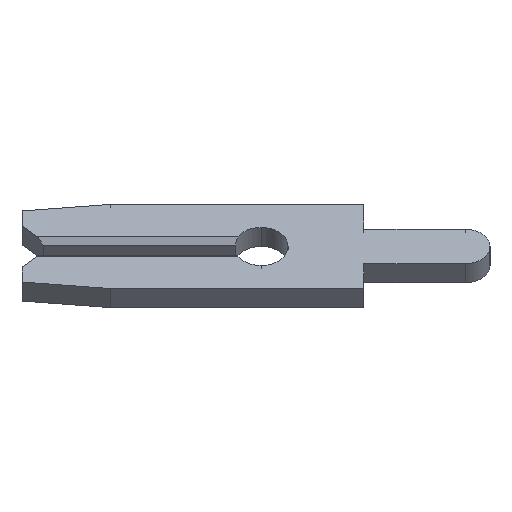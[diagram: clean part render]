
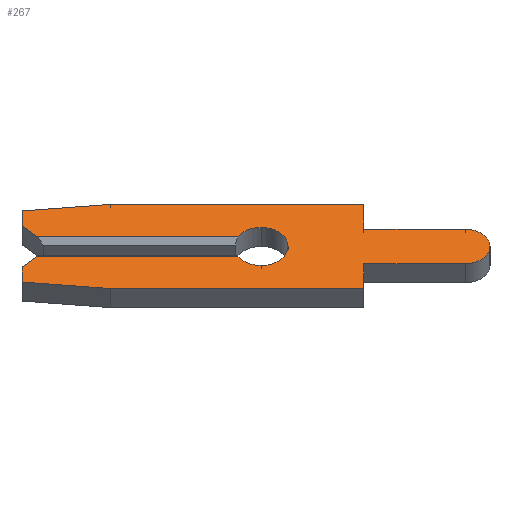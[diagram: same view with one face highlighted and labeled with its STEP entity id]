
A CAD part, left-side view. The second image highlights one B-rep face of the part: STEP entity #267.
In plain terms, the highlighted face is planar.
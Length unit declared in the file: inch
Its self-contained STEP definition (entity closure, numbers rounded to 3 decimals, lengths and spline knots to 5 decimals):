
#16 = EDGE_CURVE ( 'NONE', #715, #768, #471, .T. ) ;
#20 = DIRECTION ( 'NONE',  ( 0., 0., -1. ) ) ;
#25 = ORIENTED_EDGE ( 'NONE', *, *, #1155, .F. ) ;
#41 = CIRCLE ( 'NONE', #1211, 0.0235 ) ;
#47 = CARTESIAN_POINT ( 'NONE',  ( -0.013, 0., 0. ) ) ;
#56 = VECTOR ( 'NONE', #752, 39.37008 ) ;
#82 = ORIENTED_EDGE ( 'NONE', *, *, #520, .F. ) ;
#83 = VERTEX_POINT ( 'NONE', #694 ) ;
#90 = VERTEX_POINT ( 'NONE', #795 ) ;
#103 = VECTOR ( 'NONE', #990, 39.37008 ) ;
#115 = AXIS2_PLACEMENT_3D ( 'NONE', #521, #334, #530 ) ;
#136 = DIRECTION ( 'NONE',  ( 1., 0., 0. ) ) ;
#151 = EDGE_LOOP ( 'NONE', ( #186, #346, #287, #1049, #719, #270, #311, #524, #25, #552, #1169, #490, #344, #538, #629, #482, #82, #932 ) ) ;
#157 = EDGE_CURVE ( 'NONE', #233, #443, #610, .T. ) ;
#159 = VERTEX_POINT ( 'NONE', #923 ) ;
#168 = CIRCLE ( 'NONE', #907, 0.026 ) ;
#169 = AXIS2_PLACEMENT_3D ( 'NONE', #423, #1178, #20 ) ;
#186 = ORIENTED_EDGE ( 'NONE', *, *, #855, .T. ) ;
#187 = CARTESIAN_POINT ( 'NONE',  ( -0.013, -0.099, 0.0575 ) ) ;
#212 = CARTESIAN_POINT ( 'NONE',  ( -0.013, 0.146, -0.0575 ) ) ;
#213 = LINE ( 'NONE', #580, #922 ) ;
#221 = VERTEX_POINT ( 'NONE', #709 ) ;
#232 = DIRECTION ( 'NONE',  ( 0., -1., 0. ) ) ;
#233 = VERTEX_POINT ( 'NONE', #624 ) ;
#241 = VECTOR ( 'NONE', #620, 39.37008 ) ;
#261 = DIRECTION ( 'NONE',  ( -1., 0., 0. ) ) ;
#267 = ADVANCED_FACE ( 'NONE', ( #796 ), #823, .F. ) ;
#270 = ORIENTED_EDGE ( 'NONE', *, *, #1228, .F. ) ;
#276 = LINE ( 'NONE', #856, #56 ) ;
#287 = ORIENTED_EDGE ( 'NONE', *, *, #306, .F. ) ;
#294 = DIRECTION ( 'NONE',  ( 0., 0., 1. ) ) ;
#306 = EDGE_CURVE ( 'NONE', #369, #233, #168, .T. ) ;
#311 = ORIENTED_EDGE ( 'NONE', *, *, #755, .F. ) ;
#315 = VECTOR ( 'NONE', #906, 39.37008 ) ;
#334 = DIRECTION ( 'NONE',  ( -1., 0., 0. ) ) ;
#342 = CIRCLE ( 'NONE', #169, 0.026 ) ;
#344 = ORIENTED_EDGE ( 'NONE', *, *, #748, .F. ) ;
#346 = ORIENTED_EDGE ( 'NONE', *, *, #157, .F. ) ;
#348 = CARTESIAN_POINT ( 'NONE',  ( -0.013, 0.216, 0.013 ) ) ;
#363 = CARTESIAN_POINT ( 'NONE',  ( -0.013, 0.146, 0.0575 ) ) ;
#364 = LINE ( 'NONE', #685, #103 ) ;
#369 = VERTEX_POINT ( 'NONE', #827 ) ;
#374 = LINE ( 'NONE', #749, #789 ) ;
#379 = CARTESIAN_POINT ( 'NONE',  ( -0.013, 0.231, -0.04857 ) ) ;
#381 = DIRECTION ( 'NONE',  ( 0., 0.995, 0.105 ) ) ;
#395 = CARTESIAN_POINT ( 'NONE',  ( -0.013, -0.099, -0.0575 ) ) ;
#423 = CARTESIAN_POINT ( 'NONE',  ( -0.013, 0., 0. ) ) ;
#436 = EDGE_CURVE ( 'NONE', #810, #618, #509, .T. ) ;
#441 = EDGE_CURVE ( 'NONE', #159, #1137, #41, .T. ) ;
#443 = VERTEX_POINT ( 'NONE', #651 ) ;
#455 = DIRECTION ( 'NONE',  ( 0., -1., 0. ) ) ;
#457 = EDGE_CURVE ( 'NONE', #83, #688, #539, .T. ) ;
#467 = LINE ( 'NONE', #1205, #1192 ) ;
#471 = LINE ( 'NONE', #1003, #241 ) ;
#482 = ORIENTED_EDGE ( 'NONE', *, *, #998, .F. ) ;
#486 = CARTESIAN_POINT ( 'NONE',  ( -0.013, 0.2105, 0.0075 ) ) ;
#490 = ORIENTED_EDGE ( 'NONE', *, *, #441, .F. ) ;
#505 = VECTOR ( 'NONE', #381, 39.37008 ) ;
#509 = LINE ( 'NONE', #729, #1013 ) ;
#513 = CARTESIAN_POINT ( 'NONE',  ( -0.013, 0.231, 0.013 ) ) ;
#520 = EDGE_CURVE ( 'NONE', #1188, #90, #374, .T. ) ;
#521 = CARTESIAN_POINT ( 'NONE',  ( -0.013, 0., 0. ) ) ;
#524 = ORIENTED_EDGE ( 'NONE', *, *, #581, .F. ) ;
#530 = DIRECTION ( 'NONE',  ( 0., 0., -1. ) ) ;
#538 = ORIENTED_EDGE ( 'NONE', *, *, #1117, .F. ) ;
#539 = LINE ( 'NONE', #363, #984 ) ;
#540 = DIRECTION ( 'NONE',  ( 0., 1., 0. ) ) ;
#552 = ORIENTED_EDGE ( 'NONE', *, *, #16, .F. ) ;
#554 = VECTOR ( 'NONE', #1194, 39.37008 ) ;
#580 = CARTESIAN_POINT ( 'NONE',  ( -0.013, 0.231, -0.028 ) ) ;
#581 = EDGE_CURVE ( 'NONE', #738, #221, #645, .T. ) ;
#597 = DIRECTION ( 'NONE',  ( 0., 0.707, 0.707 ) ) ;
#610 = CIRCLE ( 'NONE', #115, 0.026 ) ;
#618 = VERTEX_POINT ( 'NONE', #949 ) ;
#620 = DIRECTION ( 'NONE',  ( 0., 0., -1. ) ) ;
#624 = CARTESIAN_POINT ( 'NONE',  ( -0.013, 0., 0.026 ) ) ;
#629 = ORIENTED_EDGE ( 'NONE', *, *, #457, .F. ) ;
#635 = CARTESIAN_POINT ( 'NONE',  ( -0.013, -0.099, 0.0575 ) ) ;
#638 = CARTESIAN_POINT ( 'NONE',  ( -0.013, -0.1975, -0.0235 ) ) ;
#645 = LINE ( 'NONE', #379, #505 ) ;
#651 = CARTESIAN_POINT ( 'NONE',  ( -0.013, 0.02252, 0.013 ) ) ;
#660 = LINE ( 'NONE', #954, #1040 ) ;
#683 = CARTESIAN_POINT ( 'NONE',  ( -0.013, -0.099, -0.0235 ) ) ;
#685 = CARTESIAN_POINT ( 'NONE',  ( -0.013, -0.099, 0.0235 ) ) ;
#688 = VERTEX_POINT ( 'NONE', #187 ) ;
#694 = CARTESIAN_POINT ( 'NONE',  ( -0.013, 0.146, 0.0575 ) ) ;
#703 = CARTESIAN_POINT ( 'NONE',  ( -0.013, 0.231, 0.04857 ) ) ;
#709 = CARTESIAN_POINT ( 'NONE',  ( -0.013, 0.231, -0.04857 ) ) ;
#715 = VERTEX_POINT ( 'NONE', #683 ) ;
#719 = ORIENTED_EDGE ( 'NONE', *, *, #436, .F. ) ;
#722 = DIRECTION ( 'NONE',  ( 0., 0., -1. ) ) ;
#727 = LINE ( 'NONE', #486, #1061 ) ;
#729 = CARTESIAN_POINT ( 'NONE',  ( -0.013, 0., -0.013 ) ) ;
#731 = DIRECTION ( 'NONE',  ( 0., 0., -1. ) ) ;
#736 = DIRECTION ( 'NONE',  ( 1., 0., 0. ) ) ;
#738 = VERTEX_POINT ( 'NONE', #212 ) ;
#746 = DIRECTION ( 'NONE',  ( 0., 0., 1. ) ) ;
#748 = EDGE_CURVE ( 'NONE', #913, #159, #364, .T. ) ;
#749 = CARTESIAN_POINT ( 'NONE',  ( -0.013, 0.231, 0.028 ) ) ;
#752 = DIRECTION ( 'NONE',  ( 0., -0.707, 0.707 ) ) ;
#755 = EDGE_CURVE ( 'NONE', #221, #1012, #213, .T. ) ;
#768 = VERTEX_POINT ( 'NONE', #395 ) ;
#770 = LINE ( 'NONE', #635, #554 ) ;
#789 = VECTOR ( 'NONE', #746, 39.37008 ) ;
#794 = LINE ( 'NONE', #513, #947 ) ;
#795 = CARTESIAN_POINT ( 'NONE',  ( -0.013, 0.231, 0.04857 ) ) ;
#796 = FACE_OUTER_BOUND ( 'NONE', #151, .T. ) ;
#797 = EDGE_CURVE ( 'NONE', #1115, #1188, #727, .T. ) ;
#810 = VERTEX_POINT ( 'NONE', #974 ) ;
#823 = PLANE ( 'NONE',  #957 ) ;
#827 = CARTESIAN_POINT ( 'NONE',  ( -0.013, 0., -0.026 ) ) ;
#831 = CARTESIAN_POINT ( 'NONE',  ( -0.013, 0., 0. ) ) ;
#855 = EDGE_CURVE ( 'NONE', #1115, #443, #794, .T. ) ;
#856 = CARTESIAN_POINT ( 'NONE',  ( -0.013, 0.2105, -0.0075 ) ) ;
#906 = DIRECTION ( 'NONE',  ( 0., -0.995, 0.105 ) ) ;
#907 = AXIS2_PLACEMENT_3D ( 'NONE', #831, #261, #731 ) ;
#913 = VERTEX_POINT ( 'NONE', #1102 ) ;
#920 = CARTESIAN_POINT ( 'NONE',  ( -0.013, 0.231, -0.028 ) ) ;
#922 = VECTOR ( 'NONE', #294, 39.37008 ) ;
#923 = CARTESIAN_POINT ( 'NONE',  ( -0.013, -0.1975, 0.0235 ) ) ;
#926 = EDGE_CURVE ( 'NONE', #618, #369, #342, .T. ) ;
#932 = ORIENTED_EDGE ( 'NONE', *, *, #797, .F. ) ;
#942 = DIRECTION ( 'NONE',  ( 0., 0., 1. ) ) ;
#947 = VECTOR ( 'NONE', #232, 39.37008 ) ;
#949 = CARTESIAN_POINT ( 'NONE',  ( -0.013, 0.02252, -0.013 ) ) ;
#954 = CARTESIAN_POINT ( 'NONE',  ( -0.013, -0.099, -0.0235 ) ) ;
#957 = AXIS2_PLACEMENT_3D ( 'NONE', #47, #136, #722 ) ;
#974 = CARTESIAN_POINT ( 'NONE',  ( -0.013, 0.216, -0.013 ) ) ;
#984 = VECTOR ( 'NONE', #455, 39.37008 ) ;
#990 = DIRECTION ( 'NONE',  ( 0., -1., 0. ) ) ;
#998 = EDGE_CURVE ( 'NONE', #90, #83, #1133, .T. ) ;
#1003 = CARTESIAN_POINT ( 'NONE',  ( -0.013, -0.099, -0.0575 ) ) ;
#1012 = VERTEX_POINT ( 'NONE', #920 ) ;
#1013 = VECTOR ( 'NONE', #1119, 39.37008 ) ;
#1019 = CARTESIAN_POINT ( 'NONE',  ( -0.013, 0.231, 0.028 ) ) ;
#1040 = VECTOR ( 'NONE', #1210, 39.37008 ) ;
#1049 = ORIENTED_EDGE ( 'NONE', *, *, #926, .F. ) ;
#1061 = VECTOR ( 'NONE', #597, 39.37008 ) ;
#1102 = CARTESIAN_POINT ( 'NONE',  ( -0.013, -0.099, 0.0235 ) ) ;
#1115 = VERTEX_POINT ( 'NONE', #348 ) ;
#1117 = EDGE_CURVE ( 'NONE', #688, #913, #770, .T. ) ;
#1119 = DIRECTION ( 'NONE',  ( 0., -1., 0. ) ) ;
#1133 = LINE ( 'NONE', #703, #315 ) ;
#1137 = VERTEX_POINT ( 'NONE', #638 ) ;
#1155 = EDGE_CURVE ( 'NONE', #768, #738, #467, .T. ) ;
#1169 = ORIENTED_EDGE ( 'NONE', *, *, #1222, .F. ) ;
#1178 = DIRECTION ( 'NONE',  ( -1., 0., 0. ) ) ;
#1188 = VERTEX_POINT ( 'NONE', #1019 ) ;
#1192 = VECTOR ( 'NONE', #540, 39.37008 ) ;
#1194 = DIRECTION ( 'NONE',  ( 0., 0., -1. ) ) ;
#1205 = CARTESIAN_POINT ( 'NONE',  ( -0.013, 0.146, -0.0575 ) ) ;
#1206 = CARTESIAN_POINT ( 'NONE',  ( -0.013, -0.1975, 0. ) ) ;
#1210 = DIRECTION ( 'NONE',  ( 0., 1., 0. ) ) ;
#1211 = AXIS2_PLACEMENT_3D ( 'NONE', #1206, #736, #942 ) ;
#1222 = EDGE_CURVE ( 'NONE', #1137, #715, #660, .T. ) ;
#1228 = EDGE_CURVE ( 'NONE', #1012, #810, #276, .T. ) ;
